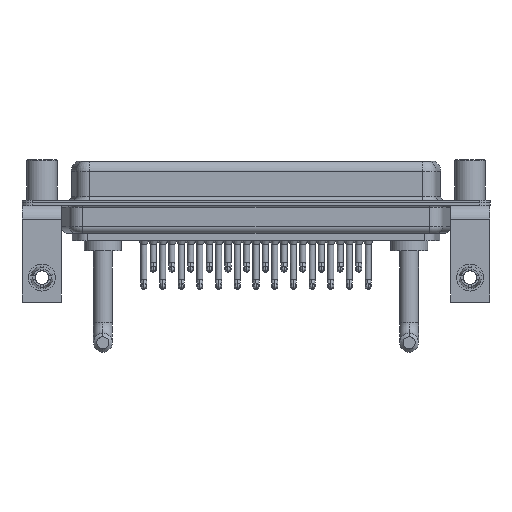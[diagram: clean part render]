
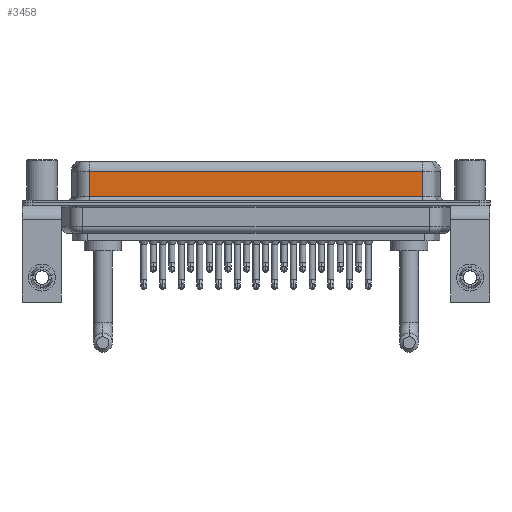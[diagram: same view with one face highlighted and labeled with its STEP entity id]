
A CAD part, front view. The second image highlights one B-rep face of the part: STEP entity #3458.
In plain terms, the highlighted planar face has unit normal (0, -1, 0).
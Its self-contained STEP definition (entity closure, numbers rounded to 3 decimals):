
#515 = VERTEX_POINT ( 'NONE', #3262 ) ;
#1590 = LINE ( 'NONE', #19237, #16816 ) ;
#1959 = CARTESIAN_POINT ( 'NONE',  ( 56.462, -3.95, 6.4 ) ) ;
#3262 = CARTESIAN_POINT ( 'NONE',  ( 7.038, -3.95, 4.65 ) ) ;
#3458 = ADVANCED_FACE ( 'NONE', ( #4103 ), #21623, .F. ) ;
#3686 = CARTESIAN_POINT ( 'NONE',  ( 7.038, -3.95, 6.4 ) ) ;
#4103 = FACE_OUTER_BOUND ( 'NONE', #14873, .T. ) ;
#4987 = CARTESIAN_POINT ( 'NONE',  ( 56.462, -3.95, 4.65 ) ) ;
#5829 = VERTEX_POINT ( 'NONE', #4987 ) ;
#8246 = LINE ( 'NONE', #19155, #24659 ) ;
#10570 = ORIENTED_EDGE ( 'NONE', *, *, #13926, .T. ) ;
#10702 = DIRECTION ( 'NONE',  ( 0., 1., 0. ) ) ;
#11946 = CARTESIAN_POINT ( 'NONE',  ( 7.038, -3.95, 0.9 ) ) ;
#12617 = CARTESIAN_POINT ( 'NONE',  ( 56.462, -3.95, 0.9 ) ) ;
#13926 = EDGE_CURVE ( 'NONE', #18218, #26755, #19150, .T. ) ;
#14873 = EDGE_LOOP ( 'NONE', ( #19476, #23717, #21483, #10570 ) ) ;
#15282 = VECTOR ( 'NONE', #19295, 1000. ) ;
#16147 = VECTOR ( 'NONE', #22697, 1000. ) ;
#16244 = LINE ( 'NONE', #3686, #16147 ) ;
#16816 = VECTOR ( 'NONE', #27851, 1000. ) ;
#16985 = EDGE_CURVE ( 'NONE', #5829, #515, #8246, .T. ) ;
#18218 = VERTEX_POINT ( 'NONE', #11946 ) ;
#18387 = EDGE_CURVE ( 'NONE', #5829, #26755, #1590, .T. ) ;
#19150 = LINE ( 'NONE', #25350, #15282 ) ;
#19155 = CARTESIAN_POINT ( 'NONE',  ( 56.462, -3.95, 4.65 ) ) ;
#19237 = CARTESIAN_POINT ( 'NONE',  ( 56.462, -3.95, 6.4 ) ) ;
#19295 = DIRECTION ( 'NONE',  ( 1., 0., 0. ) ) ;
#19476 = ORIENTED_EDGE ( 'NONE', *, *, #18387, .F. ) ;
#21483 = ORIENTED_EDGE ( 'NONE', *, *, #22737, .T. ) ;
#21623 = PLANE ( 'NONE',  #22396 ) ;
#22396 = AXIS2_PLACEMENT_3D ( 'NONE', #1959, #10702, #23348 ) ;
#22697 = DIRECTION ( 'NONE',  ( 0., 0., -1. ) ) ;
#22737 = EDGE_CURVE ( 'NONE', #515, #18218, #16244, .T. ) ;
#23348 = DIRECTION ( 'NONE',  ( 0., 0., 1. ) ) ;
#23717 = ORIENTED_EDGE ( 'NONE', *, *, #16985, .T. ) ;
#24659 = VECTOR ( 'NONE', #26048, 1000. ) ;
#25350 = CARTESIAN_POINT ( 'NONE',  ( 56.462, -3.95, 0.9 ) ) ;
#26048 = DIRECTION ( 'NONE',  ( -1., 0., 0. ) ) ;
#26755 = VERTEX_POINT ( 'NONE', #12617 ) ;
#27851 = DIRECTION ( 'NONE',  ( 0., 0., -1. ) ) ;
